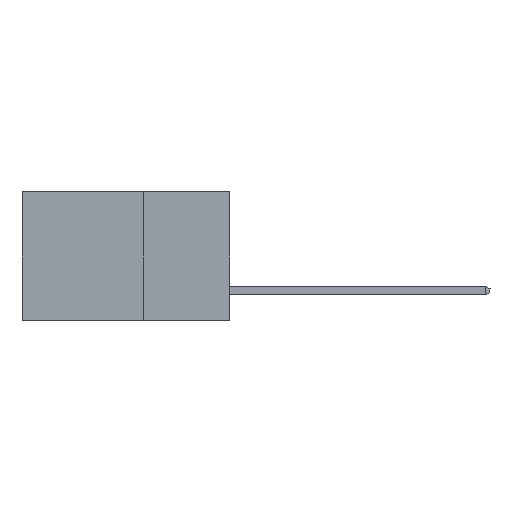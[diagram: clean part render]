
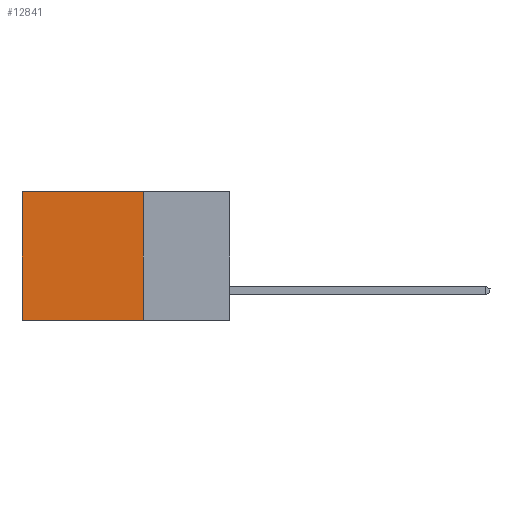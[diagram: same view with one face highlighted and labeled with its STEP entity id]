
A CAD part, left-side view. The second image highlights one B-rep face of the part: STEP entity #12841.
In plain terms, the highlighted planar face has unit normal (-1, 0, 0).
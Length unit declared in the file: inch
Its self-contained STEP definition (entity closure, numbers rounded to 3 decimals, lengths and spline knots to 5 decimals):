
#132 = CARTESIAN_POINT ( 'NONE',  ( 0.2615, 0.25, -0.37 ) ) ;
#632 = CARTESIAN_POINT ( 'NONE',  ( 0.2615, 0.25, -0.37 ) ) ;
#907 = VECTOR ( 'NONE', #6100, 39.37008 ) ;
#1382 = VERTEX_POINT ( 'NONE', #1995 ) ;
#1411 = ORIENTED_EDGE ( 'NONE', *, *, #4386, .F. ) ;
#1852 = ORIENTED_EDGE ( 'NONE', *, *, #11370, .T. ) ;
#1995 = CARTESIAN_POINT ( 'NONE',  ( 0.2615, 0.6, -0.37 ) ) ;
#2017 = EDGE_CURVE ( 'NONE', #8156, #1382, #2730, .T. ) ;
#2730 = LINE ( 'NONE', #3843, #3341 ) ;
#2879 = DIRECTION ( 'NONE',  ( 0., 1., 0. ) ) ;
#3341 = VECTOR ( 'NONE', #2879, 39.37008 ) ;
#3843 = CARTESIAN_POINT ( 'NONE',  ( 0.2615, 0.25, -0.37 ) ) ;
#4289 = VERTEX_POINT ( 'NONE', #5865 ) ;
#4321 = DIRECTION ( 'NONE',  ( 1., 0., 0. ) ) ;
#4386 = EDGE_CURVE ( 'NONE', #4289, #8156, #9904, .T. ) ;
#4474 = DIRECTION ( 'NONE',  ( 0., 0., -1. ) ) ;
#4894 = CARTESIAN_POINT ( 'NONE',  ( 0.2615, 0.6, -0.37 ) ) ;
#5811 = VECTOR ( 'NONE', #7146, 39.37008 ) ;
#5865 = CARTESIAN_POINT ( 'NONE',  ( 0.2615, 0.25, 0. ) ) ;
#6100 = DIRECTION ( 'NONE',  ( 0., 0., -1. ) ) ;
#6136 = EDGE_CURVE ( 'NONE', #12567, #1382, #7205, .T. ) ;
#6764 = VECTOR ( 'NONE', #13925, 39.37008 ) ;
#7146 = DIRECTION ( 'NONE',  ( 0., 0., -1. ) ) ;
#7205 = LINE ( 'NONE', #4894, #907 ) ;
#8112 = FACE_OUTER_BOUND ( 'NONE', #12890, .T. ) ;
#8156 = VERTEX_POINT ( 'NONE', #12044 ) ;
#9201 = LINE ( 'NONE', #14007, #6764 ) ;
#9904 = LINE ( 'NONE', #132, #5811 ) ;
#10829 = AXIS2_PLACEMENT_3D ( 'NONE', #632, #4321, #4474 ) ;
#11330 = ORIENTED_EDGE ( 'NONE', *, *, #2017, .F. ) ;
#11370 = EDGE_CURVE ( 'NONE', #4289, #12567, #9201, .T. ) ;
#11693 = ORIENTED_EDGE ( 'NONE', *, *, #6136, .T. ) ;
#12044 = CARTESIAN_POINT ( 'NONE',  ( 0.2615, 0.25, -0.37 ) ) ;
#12567 = VERTEX_POINT ( 'NONE', #13098 ) ;
#12841 = ADVANCED_FACE ( 'NONE', ( #8112 ), #14974, .F. ) ;
#12890 = EDGE_LOOP ( 'NONE', ( #11693, #11330, #1411, #1852 ) ) ;
#13098 = CARTESIAN_POINT ( 'NONE',  ( 0.2615, 0.6, 0. ) ) ;
#13925 = DIRECTION ( 'NONE',  ( 0., 1., 0. ) ) ;
#14007 = CARTESIAN_POINT ( 'NONE',  ( 0.2615, 0.25, 0. ) ) ;
#14974 = PLANE ( 'NONE',  #10829 ) ;
